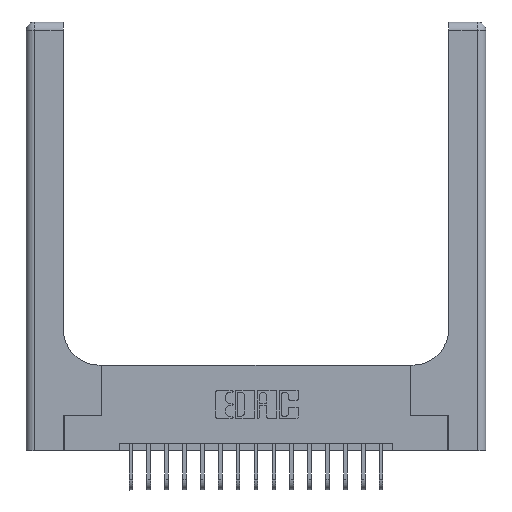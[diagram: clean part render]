
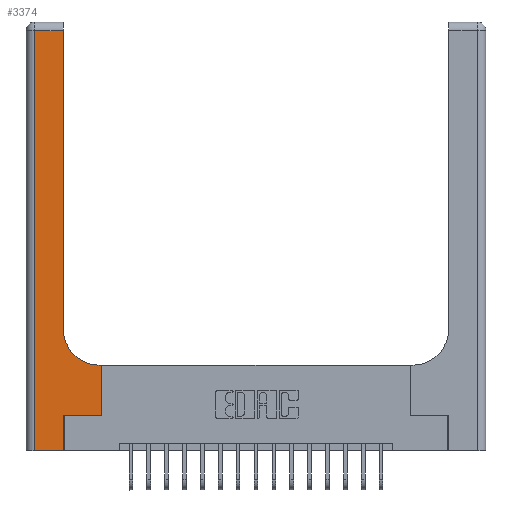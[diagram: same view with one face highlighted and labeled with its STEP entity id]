
A CAD part, top view. The second image highlights one B-rep face of the part: STEP entity #3374.
In plain terms, the highlighted planar face has unit normal (0, 0, 1).
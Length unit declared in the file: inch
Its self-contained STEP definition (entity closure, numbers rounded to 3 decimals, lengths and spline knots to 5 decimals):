
#254 = LINE ( 'NONE', #17659, #16024 ) ;
#474 = VECTOR ( 'NONE', #18399, 39.37008 ) ;
#1080 = CARTESIAN_POINT ( 'NONE',  ( 0.26, 0.85, 0.37 ) ) ;
#1373 = EDGE_CURVE ( 'NONE', #15470, #5482, #14729, .T. ) ;
#1382 = VECTOR ( 'NONE', #9391, 39.37008 ) ;
#1412 = ORIENTED_EDGE ( 'NONE', *, *, #1373, .T. ) ;
#1432 = CARTESIAN_POINT ( 'NONE',  ( 0.51, 0.6, 0.37 ) ) ;
#1939 = DIRECTION ( 'NONE',  ( 0., 0., -1. ) ) ;
#2022 = VERTEX_POINT ( 'NONE', #4477 ) ;
#2465 = AXIS2_PLACEMENT_3D ( 'NONE', #19747, #5578, #13421 ) ;
#2765 = EDGE_CURVE ( 'NONE', #11469, #3154, #6057, .T. ) ;
#3154 = VERTEX_POINT ( 'NONE', #17054 ) ;
#3311 = VECTOR ( 'NONE', #5081, 39.37008 ) ;
#3374 = ADVANCED_FACE ( 'NONE', ( #11696 ), #18149, .F. ) ;
#3655 = VECTOR ( 'NONE', #11437, 39.37008 ) ;
#4110 = VERTEX_POINT ( 'NONE', #19657 ) ;
#4356 = LINE ( 'NONE', #18806, #1382 ) ;
#4477 = CARTESIAN_POINT ( 'NONE',  ( 0.528, 0.25, 0.37 ) ) ;
#4578 = EDGE_CURVE ( 'NONE', #2022, #15470, #6206, .T. ) ;
#5047 = CARTESIAN_POINT ( 'NONE',  ( 0.51, 0.85, 0.37 ) ) ;
#5081 = DIRECTION ( 'NONE',  ( 0., 1., 0. ) ) ;
#5171 = CARTESIAN_POINT ( 'NONE',  ( 0.26, 0.6, 0.37 ) ) ;
#5221 = DIRECTION ( 'NONE',  ( 0., 1., 0. ) ) ;
#5482 = VERTEX_POINT ( 'NONE', #1432 ) ;
#5578 = DIRECTION ( 'NONE',  ( 0., 0., -1. ) ) ;
#5685 = CARTESIAN_POINT ( 'NONE',  ( 0., 2.94, 0.37 ) ) ;
#6057 = LINE ( 'NONE', #10195, #9496 ) ;
#6069 = EDGE_CURVE ( 'NONE', #4110, #2022, #8126, .T. ) ;
#6206 = LINE ( 'NONE', #6710, #18265 ) ;
#6710 = CARTESIAN_POINT ( 'NONE',  ( 0.528, 0.25, 0.37 ) ) ;
#6911 = DIRECTION ( 'NONE',  ( 0., -1., 0. ) ) ;
#7627 = EDGE_CURVE ( 'NONE', #11826, #11469, #8618, .T. ) ;
#7813 = EDGE_CURVE ( 'NONE', #3154, #9660, #4356, .T. ) ;
#8126 = LINE ( 'NONE', #14216, #19701 ) ;
#8618 = LINE ( 'NONE', #5685, #474 ) ;
#9359 = CIRCLE ( 'NONE', #17525, 0.25 ) ;
#9391 = DIRECTION ( 'NONE',  ( 1., 0., 0. ) ) ;
#9496 = VECTOR ( 'NONE', #6911, 39.37008 ) ;
#9660 = VERTEX_POINT ( 'NONE', #18683 ) ;
#10195 = CARTESIAN_POINT ( 'NONE',  ( 0.06, 3., 0.37 ) ) ;
#10578 = CARTESIAN_POINT ( 'NONE',  ( 0.26, 2.94, 0.37 ) ) ;
#11143 = CARTESIAN_POINT ( 'NONE',  ( 0.265, 0., 0.37 ) ) ;
#11179 = ORIENTED_EDGE ( 'NONE', *, *, #14728, .T. ) ;
#11437 = DIRECTION ( 'NONE',  ( -1., 0., 0. ) ) ;
#11469 = VERTEX_POINT ( 'NONE', #20216 ) ;
#11681 = EDGE_CURVE ( 'NONE', #18303, #11826, #254, .T. ) ;
#11696 = FACE_OUTER_BOUND ( 'NONE', #12827, .T. ) ;
#11826 = VERTEX_POINT ( 'NONE', #10578 ) ;
#12699 = DIRECTION ( 'NONE',  ( 1., 0., 0. ) ) ;
#12760 = ORIENTED_EDGE ( 'NONE', *, *, #2765, .T. ) ;
#12827 = EDGE_LOOP ( 'NONE', ( #14901, #19017, #12760, #15758, #19279, #14686, #18714, #1412, #11179 ) ) ;
#13034 = DIRECTION ( 'NONE',  ( 0., 1., 0. ) ) ;
#13421 = DIRECTION ( 'NONE',  ( -1., 0., 0. ) ) ;
#14216 = CARTESIAN_POINT ( 'NONE',  ( 0.265, 0.25, 0.37 ) ) ;
#14377 = LINE ( 'NONE', #11143, #3311 ) ;
#14686 = ORIENTED_EDGE ( 'NONE', *, *, #6069, .T. ) ;
#14728 = EDGE_CURVE ( 'NONE', #5482, #18303, #9359, .T. ) ;
#14729 = LINE ( 'NONE', #5171, #3655 ) ;
#14901 = ORIENTED_EDGE ( 'NONE', *, *, #11681, .T. ) ;
#15470 = VERTEX_POINT ( 'NONE', #16487 ) ;
#15758 = ORIENTED_EDGE ( 'NONE', *, *, #7813, .T. ) ;
#16024 = VECTOR ( 'NONE', #5221, 39.37008 ) ;
#16032 = DIRECTION ( 'NONE',  ( 1., 0., 0. ) ) ;
#16487 = CARTESIAN_POINT ( 'NONE',  ( 0.528, 0.6, 0.37 ) ) ;
#17054 = CARTESIAN_POINT ( 'NONE',  ( 0.06, 0., 0.37 ) ) ;
#17525 = AXIS2_PLACEMENT_3D ( 'NONE', #5047, #1939, #16032 ) ;
#17659 = CARTESIAN_POINT ( 'NONE',  ( 0.26, 3., 0.37 ) ) ;
#18149 = PLANE ( 'NONE',  #2465 ) ;
#18265 = VECTOR ( 'NONE', #13034, 39.37008 ) ;
#18303 = VERTEX_POINT ( 'NONE', #1080 ) ;
#18399 = DIRECTION ( 'NONE',  ( -1., 0., 0. ) ) ;
#18424 = EDGE_CURVE ( 'NONE', #9660, #4110, #14377, .T. ) ;
#18683 = CARTESIAN_POINT ( 'NONE',  ( 0.265, 0., 0.37 ) ) ;
#18714 = ORIENTED_EDGE ( 'NONE', *, *, #4578, .T. ) ;
#18806 = CARTESIAN_POINT ( 'NONE',  ( 0., 0., 0.37 ) ) ;
#19017 = ORIENTED_EDGE ( 'NONE', *, *, #7627, .T. ) ;
#19279 = ORIENTED_EDGE ( 'NONE', *, *, #18424, .T. ) ;
#19657 = CARTESIAN_POINT ( 'NONE',  ( 0.265, 0.25, 0.37 ) ) ;
#19701 = VECTOR ( 'NONE', #12699, 39.37008 ) ;
#19747 = CARTESIAN_POINT ( 'NONE',  ( 0., 3., 0.37 ) ) ;
#20216 = CARTESIAN_POINT ( 'NONE',  ( 0.06, 2.94, 0.37 ) ) ;
